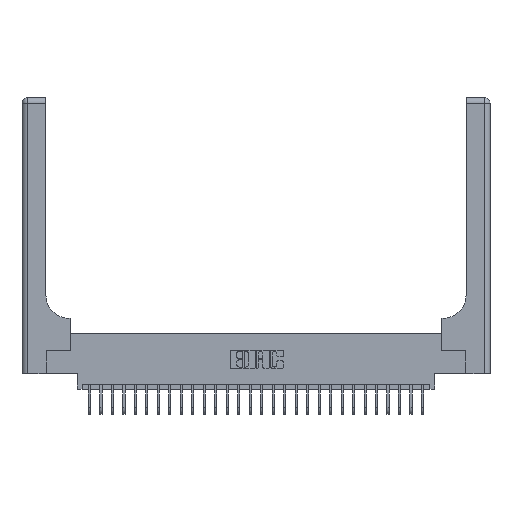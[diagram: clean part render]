
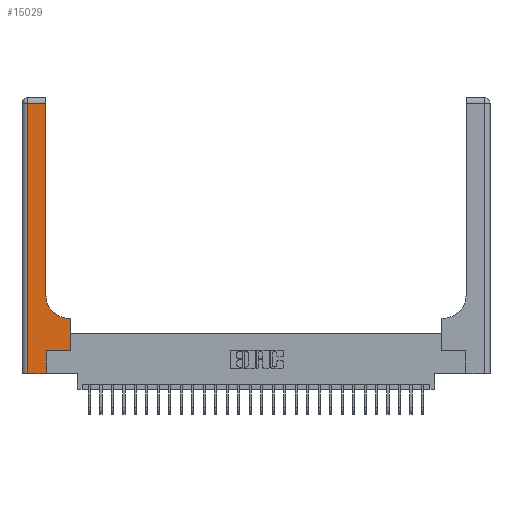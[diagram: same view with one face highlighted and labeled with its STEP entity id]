
A CAD part, top view. The second image highlights one B-rep face of the part: STEP entity #15029.
In plain terms, the highlighted planar face has unit normal (0, 0, 1).
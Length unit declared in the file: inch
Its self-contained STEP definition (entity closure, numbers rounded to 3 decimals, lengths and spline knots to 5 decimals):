
#1606 = LINE ( 'NONE', #5402, #18054 ) ;
#1907 = EDGE_CURVE ( 'NONE', #13379, #2799, #7988, .T. ) ;
#2140 = LINE ( 'NONE', #14300, #6825 ) ;
#2380 = CARTESIAN_POINT ( 'NONE',  ( 0.51, 0.85, 0.37 ) ) ;
#2385 = CARTESIAN_POINT ( 'NONE',  ( 0.528, 0.25, 0.37 ) ) ;
#2574 = ORIENTED_EDGE ( 'NONE', *, *, #11527, .T. ) ;
#2799 = VERTEX_POINT ( 'NONE', #21006 ) ;
#3013 = DIRECTION ( 'NONE',  ( -1., 0., 0. ) ) ;
#3101 = LINE ( 'NONE', #21567, #22962 ) ;
#3986 = EDGE_CURVE ( 'NONE', #14587, #22427, #7656, .T. ) ;
#3990 = AXIS2_PLACEMENT_3D ( 'NONE', #2380, #16254, #4364 ) ;
#4148 = CARTESIAN_POINT ( 'NONE',  ( 0., 2.94, 0.37 ) ) ;
#4364 = DIRECTION ( 'NONE',  ( 1., 0., 0. ) ) ;
#4417 = DIRECTION ( 'NONE',  ( 1., 0., 0. ) ) ;
#4433 = ORIENTED_EDGE ( 'NONE', *, *, #7182, .T. ) ;
#4794 = DIRECTION ( 'NONE',  ( 0., -1., 0. ) ) ;
#5275 = VERTEX_POINT ( 'NONE', #25252 ) ;
#5402 = CARTESIAN_POINT ( 'NONE',  ( 0.26, 0.6, 0.37 ) ) ;
#5477 = AXIS2_PLACEMENT_3D ( 'NONE', #12928, #14873, #3013 ) ;
#6256 = EDGE_CURVE ( 'NONE', #11705, #22454, #1606, .T. ) ;
#6825 = VECTOR ( 'NONE', #4417, 39.37008 ) ;
#7182 = EDGE_CURVE ( 'NONE', #2799, #11705, #7210, .T. ) ;
#7210 = LINE ( 'NONE', #2385, #13107 ) ;
#7487 = CARTESIAN_POINT ( 'NONE',  ( 0.26, 0.85, 0.37 ) ) ;
#7656 = LINE ( 'NONE', #17140, #22230 ) ;
#7988 = LINE ( 'NONE', #8911, #17902 ) ;
#8517 = ORIENTED_EDGE ( 'NONE', *, *, #19615, .T. ) ;
#8911 = CARTESIAN_POINT ( 'NONE',  ( 0.265, 0.25, 0.37 ) ) ;
#9336 = DIRECTION ( 'NONE',  ( -1., 0., 0. ) ) ;
#9700 = CARTESIAN_POINT ( 'NONE',  ( 0.06, 2.94, 0.37 ) ) ;
#9764 = ORIENTED_EDGE ( 'NONE', *, *, #6256, .T. ) ;
#10192 = DIRECTION ( 'NONE',  ( -1., 0., 0. ) ) ;
#10193 = EDGE_CURVE ( 'NONE', #22427, #22988, #20265, .T. ) ;
#10955 = PLANE ( 'NONE',  #5477 ) ;
#11105 = FACE_OUTER_BOUND ( 'NONE', #19134, .T. ) ;
#11272 = DIRECTION ( 'NONE',  ( 0., 1., 0. ) ) ;
#11527 = EDGE_CURVE ( 'NONE', #22988, #5275, #22093, .T. ) ;
#11705 = VERTEX_POINT ( 'NONE', #25198 ) ;
#11909 = ORIENTED_EDGE ( 'NONE', *, *, #3986, .T. ) ;
#12890 = DIRECTION ( 'NONE',  ( 1., 0., 0. ) ) ;
#12928 = CARTESIAN_POINT ( 'NONE',  ( 0., 3., 0.37 ) ) ;
#13107 = VECTOR ( 'NONE', #16259, 39.37008 ) ;
#13153 = ORIENTED_EDGE ( 'NONE', *, *, #19869, .T. ) ;
#13379 = VERTEX_POINT ( 'NONE', #21645 ) ;
#13610 = CARTESIAN_POINT ( 'NONE',  ( 0.26, 2.94, 0.37 ) ) ;
#13648 = DIRECTION ( 'NONE',  ( 0., 1., 0. ) ) ;
#14064 = CARTESIAN_POINT ( 'NONE',  ( 0.265, 0., 0.37 ) ) ;
#14300 = CARTESIAN_POINT ( 'NONE',  ( 0., 0., 0.37 ) ) ;
#14587 = VERTEX_POINT ( 'NONE', #7487 ) ;
#14873 = DIRECTION ( 'NONE',  ( 0., 0., -1. ) ) ;
#14985 = VECTOR ( 'NONE', #10192, 39.37008 ) ;
#15029 = ADVANCED_FACE ( 'NONE', ( #11105 ), #10955, .F. ) ;
#15583 = CIRCLE ( 'NONE', #3990, 0.25 ) ;
#16254 = DIRECTION ( 'NONE',  ( 0., 0., -1. ) ) ;
#16259 = DIRECTION ( 'NONE',  ( 0., 1., 0. ) ) ;
#16676 = CARTESIAN_POINT ( 'NONE',  ( 0.06, 3., 0.37 ) ) ;
#17140 = CARTESIAN_POINT ( 'NONE',  ( 0.26, 3., 0.37 ) ) ;
#17902 = VECTOR ( 'NONE', #12890, 39.37008 ) ;
#18054 = VECTOR ( 'NONE', #9336, 39.37008 ) ;
#18133 = EDGE_CURVE ( 'NONE', #22454, #14587, #15583, .T. ) ;
#18704 = VERTEX_POINT ( 'NONE', #14064 ) ;
#19026 = ORIENTED_EDGE ( 'NONE', *, *, #1907, .T. ) ;
#19134 = EDGE_LOOP ( 'NONE', ( #11909, #22463, #2574, #13153, #8517, #19026, #4433, #9764, #20260 ) ) ;
#19615 = EDGE_CURVE ( 'NONE', #18704, #13379, #3101, .T. ) ;
#19869 = EDGE_CURVE ( 'NONE', #5275, #18704, #2140, .T. ) ;
#20260 = ORIENTED_EDGE ( 'NONE', *, *, #18133, .T. ) ;
#20265 = LINE ( 'NONE', #4148, #14985 ) ;
#21006 = CARTESIAN_POINT ( 'NONE',  ( 0.528, 0.25, 0.37 ) ) ;
#21482 = VECTOR ( 'NONE', #4794, 39.37008 ) ;
#21567 = CARTESIAN_POINT ( 'NONE',  ( 0.265, 0., 0.37 ) ) ;
#21645 = CARTESIAN_POINT ( 'NONE',  ( 0.265, 0.25, 0.37 ) ) ;
#22093 = LINE ( 'NONE', #16676, #21482 ) ;
#22230 = VECTOR ( 'NONE', #11272, 39.37008 ) ;
#22427 = VERTEX_POINT ( 'NONE', #13610 ) ;
#22454 = VERTEX_POINT ( 'NONE', #25596 ) ;
#22463 = ORIENTED_EDGE ( 'NONE', *, *, #10193, .T. ) ;
#22962 = VECTOR ( 'NONE', #13648, 39.37008 ) ;
#22988 = VERTEX_POINT ( 'NONE', #9700 ) ;
#25198 = CARTESIAN_POINT ( 'NONE',  ( 0.528, 0.6, 0.37 ) ) ;
#25252 = CARTESIAN_POINT ( 'NONE',  ( 0.06, 0., 0.37 ) ) ;
#25596 = CARTESIAN_POINT ( 'NONE',  ( 0.51, 0.6, 0.37 ) ) ;
